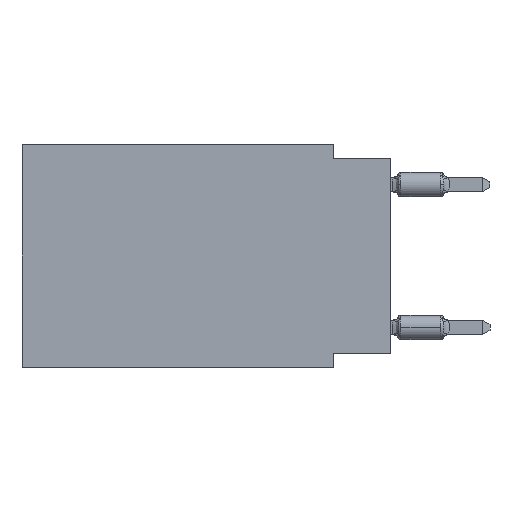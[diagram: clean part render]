
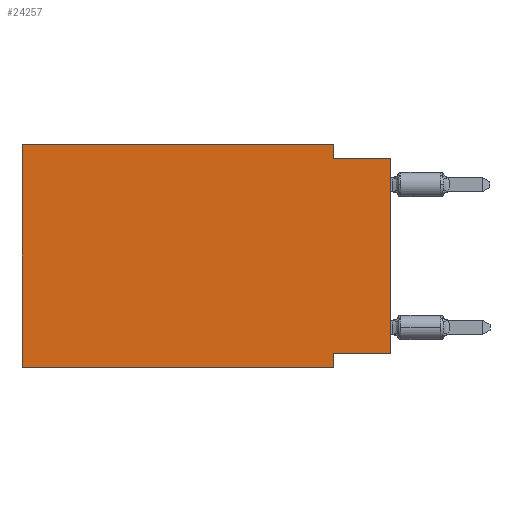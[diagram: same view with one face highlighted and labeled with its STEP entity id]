
A CAD part, left-side view. The second image highlights one B-rep face of the part: STEP entity #24257.
In plain terms, the highlighted planar face has unit normal (-1, 0, 0).
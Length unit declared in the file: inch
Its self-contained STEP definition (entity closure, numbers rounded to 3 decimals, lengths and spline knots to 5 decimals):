
#367 = CARTESIAN_POINT ( 'NONE',  ( 0., 0.645, -0.39 ) ) ;
#458 = LINE ( 'NONE', #4746, #1984 ) ;
#963 = CARTESIAN_POINT ( 'NONE',  ( 0., 0.1, -0.025 ) ) ;
#971 = DIRECTION ( 'NONE',  ( 0., 0., 1. ) ) ;
#1908 = EDGE_CURVE ( 'NONE', #15670, #5211, #458, .T. ) ;
#1984 = VECTOR ( 'NONE', #971, 39.37008 ) ;
#2055 = VECTOR ( 'NONE', #5721, 39.37008 ) ;
#2901 = EDGE_CURVE ( 'NONE', #20674, #15770, #24084, .T. ) ;
#3382 = EDGE_LOOP ( 'NONE', ( #20968, #11198, #24513, #6469, #10784, #9912, #4580, #9786 ) ) ;
#4018 = EDGE_CURVE ( 'NONE', #15670, #7347, #9766, .T. ) ;
#4388 = VECTOR ( 'NONE', #16142, 39.37008 ) ;
#4580 = ORIENTED_EDGE ( 'NONE', *, *, #14382, .F. ) ;
#4613 = EDGE_CURVE ( 'NONE', #20674, #23532, #18063, .T. ) ;
#4746 = CARTESIAN_POINT ( 'NONE',  ( 0., 0., 0. ) ) ;
#4889 = VECTOR ( 'NONE', #5291, 39.37008 ) ;
#5211 = VERTEX_POINT ( 'NONE', #13453 ) ;
#5291 = DIRECTION ( 'NONE',  ( 0., -1., 0. ) ) ;
#5388 = PLANE ( 'NONE',  #7153 ) ;
#5721 = DIRECTION ( 'NONE',  ( 0., 1., 0. ) ) ;
#5806 = LINE ( 'NONE', #23145, #4889 ) ;
#6126 = LINE ( 'NONE', #10274, #4388 ) ;
#6359 = DIRECTION ( 'NONE',  ( 0., -1., 0. ) ) ;
#6469 = ORIENTED_EDGE ( 'NONE', *, *, #10522, .F. ) ;
#7153 = AXIS2_PLACEMENT_3D ( 'NONE', #13336, #15411, #11389 ) ;
#7347 = VERTEX_POINT ( 'NONE', #25650 ) ;
#8259 = VECTOR ( 'NONE', #12478, 39.37008 ) ;
#8372 = VERTEX_POINT ( 'NONE', #20689 ) ;
#9766 = LINE ( 'NONE', #19925, #2055 ) ;
#9786 = ORIENTED_EDGE ( 'NONE', *, *, #4018, .F. ) ;
#9912 = ORIENTED_EDGE ( 'NONE', *, *, #2901, .T. ) ;
#10274 = CARTESIAN_POINT ( 'NONE',  ( 0., 0.1, 0. ) ) ;
#10355 = CARTESIAN_POINT ( 'NONE',  ( 0., 0.645, 0. ) ) ;
#10384 = CARTESIAN_POINT ( 'NONE',  ( 0., 0.645, 0. ) ) ;
#10522 = EDGE_CURVE ( 'NONE', #23532, #8372, #13836, .T. ) ;
#10784 = ORIENTED_EDGE ( 'NONE', *, *, #4613, .F. ) ;
#11198 = ORIENTED_EDGE ( 'NONE', *, *, #17246, .F. ) ;
#11389 = DIRECTION ( 'NONE',  ( 0., 0., -1. ) ) ;
#12009 = CARTESIAN_POINT ( 'NONE',  ( 0., 0.645, -0.39 ) ) ;
#12478 = DIRECTION ( 'NONE',  ( 0., -1., 0. ) ) ;
#12790 = CARTESIAN_POINT ( 'NONE',  ( 0., 0.1, -0.39 ) ) ;
#13310 = VECTOR ( 'NONE', #18183, 39.37008 ) ;
#13336 = CARTESIAN_POINT ( 'NONE',  ( 0., 0.645, 0. ) ) ;
#13453 = CARTESIAN_POINT ( 'NONE',  ( 0., 0., -0.025 ) ) ;
#13836 = LINE ( 'NONE', #10384, #24700 ) ;
#14382 = EDGE_CURVE ( 'NONE', #7347, #15770, #22544, .T. ) ;
#14665 = EDGE_CURVE ( 'NONE', #8372, #22887, #6126, .T. ) ;
#15411 = DIRECTION ( 'NONE',  ( 1., 0., 0. ) ) ;
#15541 = FACE_OUTER_BOUND ( 'NONE', #3382, .T. ) ;
#15670 = VERTEX_POINT ( 'NONE', #16938 ) ;
#15770 = VERTEX_POINT ( 'NONE', #23470 ) ;
#16142 = DIRECTION ( 'NONE',  ( 0., 0., -1. ) ) ;
#16938 = CARTESIAN_POINT ( 'NONE',  ( 0., 0., -0.365 ) ) ;
#17246 = EDGE_CURVE ( 'NONE', #22887, #5211, #5806, .T. ) ;
#18063 = LINE ( 'NONE', #10355, #13310 ) ;
#18183 = DIRECTION ( 'NONE',  ( 0., 0., 1. ) ) ;
#19283 = CARTESIAN_POINT ( 'NONE',  ( 0., 0.645, 0. ) ) ;
#19925 = CARTESIAN_POINT ( 'NONE',  ( 0., 0., -0.365 ) ) ;
#20674 = VERTEX_POINT ( 'NONE', #12009 ) ;
#20689 = CARTESIAN_POINT ( 'NONE',  ( 0., 0.1, 0. ) ) ;
#20968 = ORIENTED_EDGE ( 'NONE', *, *, #1908, .T. ) ;
#20988 = DIRECTION ( 'NONE',  ( 0., 0., -1. ) ) ;
#22544 = LINE ( 'NONE', #12790, #23537 ) ;
#22887 = VERTEX_POINT ( 'NONE', #963 ) ;
#23145 = CARTESIAN_POINT ( 'NONE',  ( 0., 0., -0.025 ) ) ;
#23470 = CARTESIAN_POINT ( 'NONE',  ( 0., 0.1, -0.39 ) ) ;
#23532 = VERTEX_POINT ( 'NONE', #19283 ) ;
#23537 = VECTOR ( 'NONE', #20988, 39.37008 ) ;
#24084 = LINE ( 'NONE', #367, #8259 ) ;
#24257 = ADVANCED_FACE ( 'NONE', ( #15541 ), #5388, .F. ) ;
#24513 = ORIENTED_EDGE ( 'NONE', *, *, #14665, .F. ) ;
#24700 = VECTOR ( 'NONE', #6359, 39.37008 ) ;
#25650 = CARTESIAN_POINT ( 'NONE',  ( 0., 0.1, -0.365 ) ) ;
